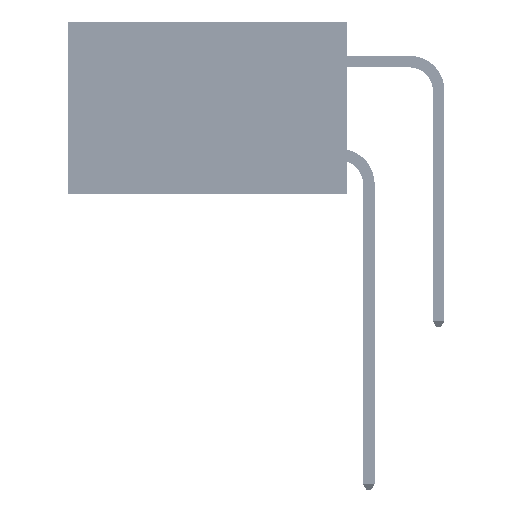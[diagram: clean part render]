
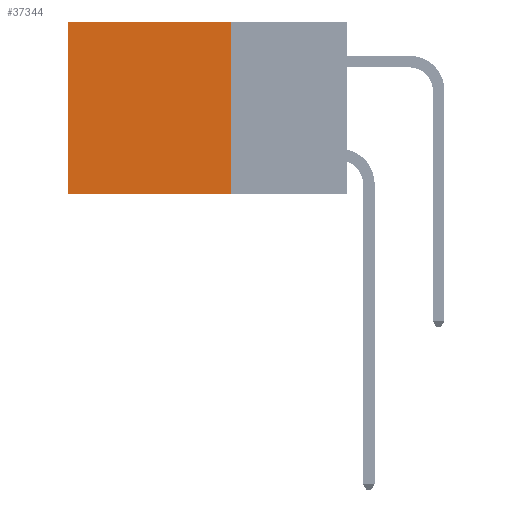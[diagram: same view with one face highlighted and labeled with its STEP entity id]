
A CAD part, left-side view. The second image highlights one B-rep face of the part: STEP entity #37344.
In plain terms, the highlighted planar face has unit normal (-1, 0, 0).
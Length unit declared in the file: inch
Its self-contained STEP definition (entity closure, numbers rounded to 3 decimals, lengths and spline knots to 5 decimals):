
#852 = CARTESIAN_POINT ( 'NONE',  ( 0.2875, 0.25, 0. ) ) ;
#932 = CARTESIAN_POINT ( 'NONE',  ( 0.2875, 0.25, 0. ) ) ;
#5598 = VERTEX_POINT ( 'NONE', #24368 ) ;
#5638 = LINE ( 'NONE', #21013, #13401 ) ;
#7700 = VERTEX_POINT ( 'NONE', #12352 ) ;
#8719 = PLANE ( 'NONE',  #41255 ) ;
#9412 = ORIENTED_EDGE ( 'NONE', *, *, #25187, .F. ) ;
#10545 = ORIENTED_EDGE ( 'NONE', *, *, #42236, .F. ) ;
#11995 = VERTEX_POINT ( 'NONE', #44547 ) ;
#12352 = CARTESIAN_POINT ( 'NONE',  ( 0.2875, 0.25, -0.37 ) ) ;
#12830 = DIRECTION ( 'NONE',  ( 1., 0., 0. ) ) ;
#13227 = ORIENTED_EDGE ( 'NONE', *, *, #32329, .T. ) ;
#13401 = VECTOR ( 'NONE', #27348, 39.37008 ) ;
#17947 = CARTESIAN_POINT ( 'NONE',  ( 0.2875, 0.25, 0. ) ) ;
#19114 = LINE ( 'NONE', #852, #29217 ) ;
#19367 = DIRECTION ( 'NONE',  ( 0., 0., -1. ) ) ;
#21013 = CARTESIAN_POINT ( 'NONE',  ( 0.2875, 0.25, -0.37 ) ) ;
#21360 = DIRECTION ( 'NONE',  ( 0., 1., 0. ) ) ;
#22380 = EDGE_LOOP ( 'NONE', ( #13227, #10545, #9412, #35404 ) ) ;
#22399 = VECTOR ( 'NONE', #26690, 39.37008 ) ;
#24368 = CARTESIAN_POINT ( 'NONE',  ( 0.2875, 0.6, 0. ) ) ;
#25187 = EDGE_CURVE ( 'NONE', #11995, #7700, #19114, .T. ) ;
#26232 = LINE ( 'NONE', #33772, #22399 ) ;
#26690 = DIRECTION ( 'NONE',  ( 0., 0., -1. ) ) ;
#27348 = DIRECTION ( 'NONE',  ( 0., 1., 0. ) ) ;
#29217 = VECTOR ( 'NONE', #19367, 39.37008 ) ;
#30651 = DIRECTION ( 'NONE',  ( 0., 0., -1. ) ) ;
#32329 = EDGE_CURVE ( 'NONE', #5598, #36020, #26232, .T. ) ;
#33152 = VECTOR ( 'NONE', #21360, 39.37008 ) ;
#33772 = CARTESIAN_POINT ( 'NONE',  ( 0.2875, 0.6, 0. ) ) ;
#35404 = ORIENTED_EDGE ( 'NONE', *, *, #46741, .T. ) ;
#36020 = VERTEX_POINT ( 'NONE', #45718 ) ;
#37344 = ADVANCED_FACE ( 'NONE', ( #42074 ), #8719, .F. ) ;
#39849 = LINE ( 'NONE', #17947, #33152 ) ;
#41255 = AXIS2_PLACEMENT_3D ( 'NONE', #932, #12830, #30651 ) ;
#42074 = FACE_OUTER_BOUND ( 'NONE', #22380, .T. ) ;
#42236 = EDGE_CURVE ( 'NONE', #7700, #36020, #5638, .T. ) ;
#44547 = CARTESIAN_POINT ( 'NONE',  ( 0.2875, 0.25, 0. ) ) ;
#45718 = CARTESIAN_POINT ( 'NONE',  ( 0.2875, 0.6, -0.37 ) ) ;
#46741 = EDGE_CURVE ( 'NONE', #11995, #5598, #39849, .T. ) ;
